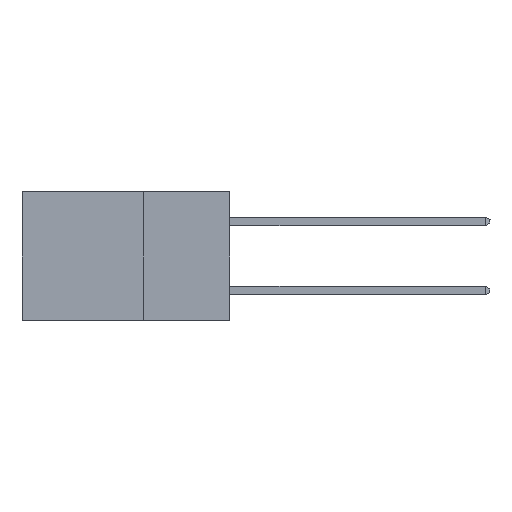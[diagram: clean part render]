
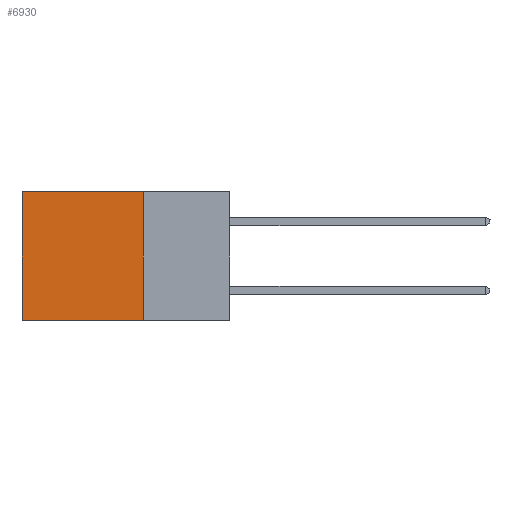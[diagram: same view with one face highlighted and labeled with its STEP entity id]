
A CAD part, left-side view. The second image highlights one B-rep face of the part: STEP entity #6930.
In plain terms, the highlighted planar face has unit normal (-1, 0, 0).
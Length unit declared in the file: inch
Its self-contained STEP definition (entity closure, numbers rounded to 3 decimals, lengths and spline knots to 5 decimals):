
#60 = CARTESIAN_POINT ( 'NONE',  ( 0.2615, 0.6, 0. ) ) ;
#332 = CARTESIAN_POINT ( 'NONE',  ( 0.2615, 0.25, -0.37 ) ) ;
#562 = EDGE_CURVE ( 'NONE', #1274, #10453, #9755, .T. ) ;
#829 = VECTOR ( 'NONE', #1176, 39.37008 ) ;
#1176 = DIRECTION ( 'NONE',  ( 0., 0., -1. ) ) ;
#1274 = VERTEX_POINT ( 'NONE', #332 ) ;
#1373 = PLANE ( 'NONE',  #2613 ) ;
#1408 = VECTOR ( 'NONE', #1480, 39.37008 ) ;
#1480 = DIRECTION ( 'NONE',  ( 0., 1., 0. ) ) ;
#1624 = ORIENTED_EDGE ( 'NONE', *, *, #3099, .F. ) ;
#1688 = CARTESIAN_POINT ( 'NONE',  ( 0.2615, 0.25, 0. ) ) ;
#2129 = ORIENTED_EDGE ( 'NONE', *, *, #4739, .T. ) ;
#2613 = AXIS2_PLACEMENT_3D ( 'NONE', #4212, #7903, #5064 ) ;
#2638 = LINE ( 'NONE', #3667, #829 ) ;
#2668 = EDGE_LOOP ( 'NONE', ( #11162, #11746, #1624, #2129 ) ) ;
#3031 = CARTESIAN_POINT ( 'NONE',  ( 0.2615, 0.6, -0.37 ) ) ;
#3033 = DIRECTION ( 'NONE',  ( 0., 1., 0. ) ) ;
#3099 = EDGE_CURVE ( 'NONE', #4930, #1274, #2638, .T. ) ;
#3667 = CARTESIAN_POINT ( 'NONE',  ( 0.2615, 0.25, -0.37 ) ) ;
#3710 = EDGE_CURVE ( 'NONE', #6347, #10453, #6235, .T. ) ;
#4212 = CARTESIAN_POINT ( 'NONE',  ( 0.2615, 0.25, -0.37 ) ) ;
#4739 = EDGE_CURVE ( 'NONE', #4930, #6347, #9631, .T. ) ;
#4930 = VERTEX_POINT ( 'NONE', #1688 ) ;
#5064 = DIRECTION ( 'NONE',  ( 0., 0., -1. ) ) ;
#5245 = CARTESIAN_POINT ( 'NONE',  ( 0.2615, 0.6, -0.37 ) ) ;
#5322 = DIRECTION ( 'NONE',  ( 0., 0., -1. ) ) ;
#5967 = FACE_OUTER_BOUND ( 'NONE', #2668, .T. ) ;
#6212 = VECTOR ( 'NONE', #5322, 39.37008 ) ;
#6235 = LINE ( 'NONE', #3031, #6212 ) ;
#6347 = VERTEX_POINT ( 'NONE', #60 ) ;
#6751 = VECTOR ( 'NONE', #3033, 39.37008 ) ;
#6930 = ADVANCED_FACE ( 'NONE', ( #5967 ), #1373, .F. ) ;
#7903 = DIRECTION ( 'NONE',  ( 1., 0., 0. ) ) ;
#8545 = CARTESIAN_POINT ( 'NONE',  ( 0.2615, 0.25, 0. ) ) ;
#9631 = LINE ( 'NONE', #8545, #6751 ) ;
#9755 = LINE ( 'NONE', #11631, #1408 ) ;
#10453 = VERTEX_POINT ( 'NONE', #5245 ) ;
#11162 = ORIENTED_EDGE ( 'NONE', *, *, #3710, .T. ) ;
#11631 = CARTESIAN_POINT ( 'NONE',  ( 0.2615, 0.25, -0.37 ) ) ;
#11746 = ORIENTED_EDGE ( 'NONE', *, *, #562, .F. ) ;
